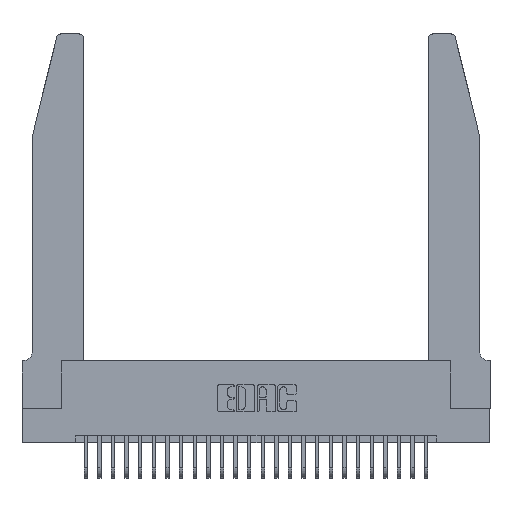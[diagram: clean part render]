
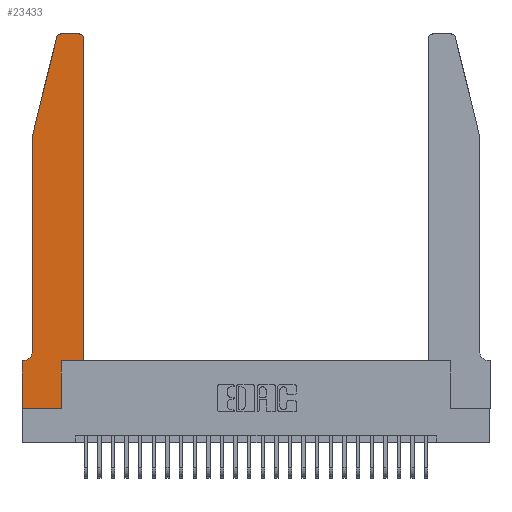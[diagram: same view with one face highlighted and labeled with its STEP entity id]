
A CAD part, top view. The second image highlights one B-rep face of the part: STEP entity #23433.
In plain terms, the highlighted planar face has unit normal (0, 0, 1).
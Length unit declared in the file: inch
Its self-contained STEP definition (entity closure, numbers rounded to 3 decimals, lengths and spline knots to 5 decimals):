
#55 = CARTESIAN_POINT ( 'NONE',  ( 0.0755, 2., 0.37 ) ) ;
#78 = DIRECTION ( 'NONE',  ( 0., -1., 0. ) ) ;
#178 = VERTEX_POINT ( 'NONE', #17069 ) ;
#266 = VECTOR ( 'NONE', #7564, 39.37008 ) ;
#944 = VECTOR ( 'NONE', #26223, 39.37008 ) ;
#1480 = ORIENTED_EDGE ( 'NONE', *, *, #22524, .T. ) ;
#1626 = ORIENTED_EDGE ( 'NONE', *, *, #17133, .T. ) ;
#2201 = LINE ( 'NONE', #17350, #6443 ) ;
#2232 = DIRECTION ( 'NONE',  ( -0.239, -0.971, 0. ) ) ;
#3398 = CARTESIAN_POINT ( 'NONE',  ( 0.4505, 0.35, 0.37 ) ) ;
#3494 = ORIENTED_EDGE ( 'NONE', *, *, #18141, .T. ) ;
#3664 = LINE ( 'NONE', #55, #19403 ) ;
#4052 = EDGE_CURVE ( 'NONE', #10526, #8417, #21478, .T. ) ;
#4095 = CARTESIAN_POINT ( 'NONE',  ( 0.4505, 0.35, 0.37 ) ) ;
#4255 = VERTEX_POINT ( 'NONE', #11020 ) ;
#4637 = VECTOR ( 'NONE', #15169, 39.37008 ) ;
#4659 = AXIS2_PLACEMENT_3D ( 'NONE', #21206, #8988, #23225 ) ;
#4796 = ORIENTED_EDGE ( 'NONE', *, *, #16415, .T. ) ;
#5649 = CARTESIAN_POINT ( 'NONE',  ( 0., 0.35, 0.37 ) ) ;
#6036 = LINE ( 'NONE', #14980, #15632 ) ;
#6169 = CARTESIAN_POINT ( 'NONE',  ( 0.284, 2.72, 0.37 ) ) ;
#6443 = VECTOR ( 'NONE', #25438, 39.37008 ) ;
#6601 = CARTESIAN_POINT ( 'NONE',  ( 0.0055, 0.35, 0.37 ) ) ;
#6890 = ORIENTED_EDGE ( 'NONE', *, *, #18178, .T. ) ;
#7170 = LINE ( 'NONE', #21832, #266 ) ;
#7197 = VECTOR ( 'NONE', #24176, 39.37008 ) ;
#7564 = DIRECTION ( 'NONE',  ( 1., 0., 0. ) ) ;
#7678 = DIRECTION ( 'NONE',  ( 0., 0., 1. ) ) ;
#7830 = CIRCLE ( 'NONE', #12186, 0.03 ) ;
#7980 = CIRCLE ( 'NONE', #22011, 0.03 ) ;
#8024 = EDGE_LOOP ( 'NONE', ( #1480, #4796, #1626, #18185, #24472, #22279, #25267, #15476, #3494, #18473, #10190, #6890 ) ) ;
#8200 = DIRECTION ( 'NONE',  ( 1., 0., 0. ) ) ;
#8417 = VERTEX_POINT ( 'NONE', #11211 ) ;
#8988 = DIRECTION ( 'NONE',  ( 0., 0., -1. ) ) ;
#9091 = CARTESIAN_POINT ( 'NONE',  ( 0.0755, 0.42, 0.37 ) ) ;
#10121 = CARTESIAN_POINT ( 'NONE',  ( 0.2865, 0., 0.37 ) ) ;
#10190 = ORIENTED_EDGE ( 'NONE', *, *, #25393, .T. ) ;
#10526 = VERTEX_POINT ( 'NONE', #16372 ) ;
#11020 = CARTESIAN_POINT ( 'NONE',  ( 0.4505, 2.72, 0.37 ) ) ;
#11211 = CARTESIAN_POINT ( 'NONE',  ( 0., 0., 0.37 ) ) ;
#11506 = CIRCLE ( 'NONE', #4659, 0.07 ) ;
#11699 = EDGE_CURVE ( 'NONE', #18541, #15194, #16866, .T. ) ;
#12186 = AXIS2_PLACEMENT_3D ( 'NONE', #12219, #26357, #14259 ) ;
#12219 = CARTESIAN_POINT ( 'NONE',  ( 0.4205, 2.72, 0.37 ) ) ;
#12660 = LINE ( 'NONE', #14078, #7197 ) ;
#13279 = CARTESIAN_POINT ( 'NONE',  ( 0.2865, 0.35, 0.37 ) ) ;
#13374 = EDGE_CURVE ( 'NONE', #8417, #17002, #7170, .T. ) ;
#14078 = CARTESIAN_POINT ( 'NONE',  ( 0.2865, 0.35, 0.37 ) ) ;
#14161 = VECTOR ( 'NONE', #78, 39.37008 ) ;
#14259 = DIRECTION ( 'NONE',  ( 1., 0., 0. ) ) ;
#14481 = EDGE_CURVE ( 'NONE', #15996, #10526, #18040, .T. ) ;
#14591 = CARTESIAN_POINT ( 'NONE',  ( 0., 0., 0.37 ) ) ;
#14980 = CARTESIAN_POINT ( 'NONE',  ( 0.2605, 2.75, 0.37 ) ) ;
#15169 = DIRECTION ( 'NONE',  ( 0., -1., 0. ) ) ;
#15194 = VERTEX_POINT ( 'NONE', #4095 ) ;
#15476 = ORIENTED_EDGE ( 'NONE', *, *, #13374, .T. ) ;
#15632 = VECTOR ( 'NONE', #25133, 39.37008 ) ;
#15996 = VERTEX_POINT ( 'NONE', #6601 ) ;
#16233 = VECTOR ( 'NONE', #19823, 39.37008 ) ;
#16372 = CARTESIAN_POINT ( 'NONE',  ( 0., 0.35, 0.37 ) ) ;
#16415 = EDGE_CURVE ( 'NONE', #20308, #178, #7980, .T. ) ;
#16491 = FACE_OUTER_BOUND ( 'NONE', #8024, .T. ) ;
#16725 = VERTEX_POINT ( 'NONE', #9091 ) ;
#16732 = AXIS2_PLACEMENT_3D ( 'NONE', #5649, #7678, #21932 ) ;
#16866 = LINE ( 'NONE', #3398, #16233 ) ;
#17002 = VERTEX_POINT ( 'NONE', #10121 ) ;
#17069 = CARTESIAN_POINT ( 'NONE',  ( 0.25487, 2.72718, 0.37 ) ) ;
#17133 = EDGE_CURVE ( 'NONE', #178, #18118, #3664, .T. ) ;
#17222 = CARTESIAN_POINT ( 'NONE',  ( 0.0755, 2., 0.37 ) ) ;
#17350 = CARTESIAN_POINT ( 'NONE',  ( 0.4505, 0.35, 0.37 ) ) ;
#17818 = EDGE_CURVE ( 'NONE', #18118, #16725, #20320, .T. ) ;
#17901 = PLANE ( 'NONE',  #16732 ) ;
#18040 = LINE ( 'NONE', #24212, #944 ) ;
#18118 = VERTEX_POINT ( 'NONE', #24093 ) ;
#18141 = EDGE_CURVE ( 'NONE', #17002, #18541, #12660, .T. ) ;
#18178 = EDGE_CURVE ( 'NONE', #4255, #26267, #7830, .T. ) ;
#18185 = ORIENTED_EDGE ( 'NONE', *, *, #17818, .T. ) ;
#18473 = ORIENTED_EDGE ( 'NONE', *, *, #11699, .T. ) ;
#18541 = VERTEX_POINT ( 'NONE', #13279 ) ;
#19167 = CARTESIAN_POINT ( 'NONE',  ( 0.284, 2.75, 0.37 ) ) ;
#19403 = VECTOR ( 'NONE', #2232, 39.37008 ) ;
#19823 = DIRECTION ( 'NONE',  ( 1., 0., 0. ) ) ;
#20308 = VERTEX_POINT ( 'NONE', #19167 ) ;
#20320 = LINE ( 'NONE', #17222, #4637 ) ;
#20439 = DIRECTION ( 'NONE',  ( 0., 0., 1. ) ) ;
#21206 = CARTESIAN_POINT ( 'NONE',  ( 0.0055, 0.42, 0.37 ) ) ;
#21478 = LINE ( 'NONE', #14591, #14161 ) ;
#21832 = CARTESIAN_POINT ( 'NONE',  ( 0., 0., 0.37 ) ) ;
#21932 = DIRECTION ( 'NONE',  ( 1., 0., 0. ) ) ;
#22011 = AXIS2_PLACEMENT_3D ( 'NONE', #6169, #20439, #8200 ) ;
#22023 = EDGE_CURVE ( 'NONE', #16725, #15996, #11506, .T. ) ;
#22279 = ORIENTED_EDGE ( 'NONE', *, *, #14481, .T. ) ;
#22524 = EDGE_CURVE ( 'NONE', #26267, #20308, #6036, .T. ) ;
#23225 = DIRECTION ( 'NONE',  ( -1., 0., 0. ) ) ;
#23433 = ADVANCED_FACE ( 'NONE', ( #16491 ), #17901, .T. ) ;
#24093 = CARTESIAN_POINT ( 'NONE',  ( 0.0755, 2., 0.37 ) ) ;
#24176 = DIRECTION ( 'NONE',  ( 0., 1., 0. ) ) ;
#24212 = CARTESIAN_POINT ( 'NONE',  ( 0.0755, 0.35, 0.37 ) ) ;
#24472 = ORIENTED_EDGE ( 'NONE', *, *, #22023, .T. ) ;
#25133 = DIRECTION ( 'NONE',  ( -1., 0., 0. ) ) ;
#25267 = ORIENTED_EDGE ( 'NONE', *, *, #4052, .T. ) ;
#25393 = EDGE_CURVE ( 'NONE', #15194, #4255, #2201, .T. ) ;
#25438 = DIRECTION ( 'NONE',  ( 0., 1., 0. ) ) ;
#26223 = DIRECTION ( 'NONE',  ( -1., 0., 0. ) ) ;
#26267 = VERTEX_POINT ( 'NONE', #26544 ) ;
#26357 = DIRECTION ( 'NONE',  ( 0., 0., 1. ) ) ;
#26544 = CARTESIAN_POINT ( 'NONE',  ( 0.4205, 2.75, 0.37 ) ) ;
